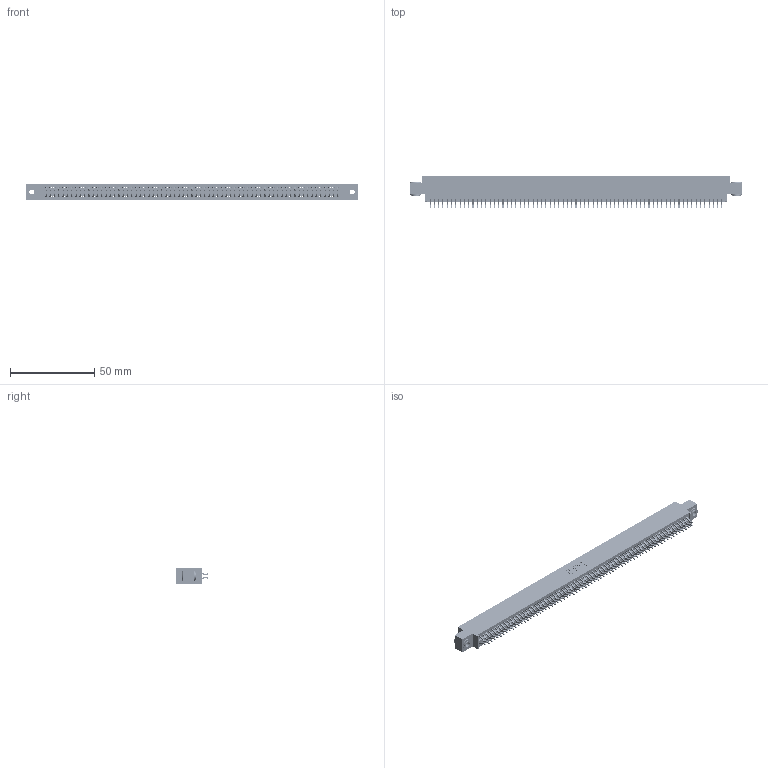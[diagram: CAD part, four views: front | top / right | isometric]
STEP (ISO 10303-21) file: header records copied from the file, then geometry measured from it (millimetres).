
FILE_DESCRIPTION (( 'STEP AP203' ), '1' );
FILE_NAME ('345-138-556-803.STEP', '2019-11-08T17:16:33', ( '' ), ( '' ), 'SwSTEP 2.0', 'SolidWorks 2016', '' );
FILE_SCHEMA (( 'CONFIG_CONTROL_DESIGN' ));
Length unit declared in the file: inch
Products named in the file (4): 345 Part_0.170 Offset - 0.156 Dia-TH; 345-292-001_556 Tail; 345-138-556-803; 345-250-002_345-250-002-102
Assembly tree (141 placements, depth 2):
  345-138-556-803
    345 Part_0.170 Offset - 0.156 Dia-TH
    345-292-001_556 Tail  x138
    345-250-002_345-250-002-102  x2
Bounding box: 196.47 x 19.24 x 9.4 mm (x, y, z)
Volume: 19236.4 mm3; surface area: 29185.1 mm2
Topology: 141 solids, 141 shells, 7896 faces, 23475 edges, 15462 vertices
Faces by surface type: plane 5200, cylinder 2688, cone 8
Entity records: 51506 total; most frequent: CARTESIAN_POINT 8599, ORIENTED_EDGE 8514, DIRECTION 7567, EDGE_CURVE 4257, VECTOR 3817, LINE 3817, VERTEX_POINT 2834, AXIS2_PLACEMENT_3D 1875
